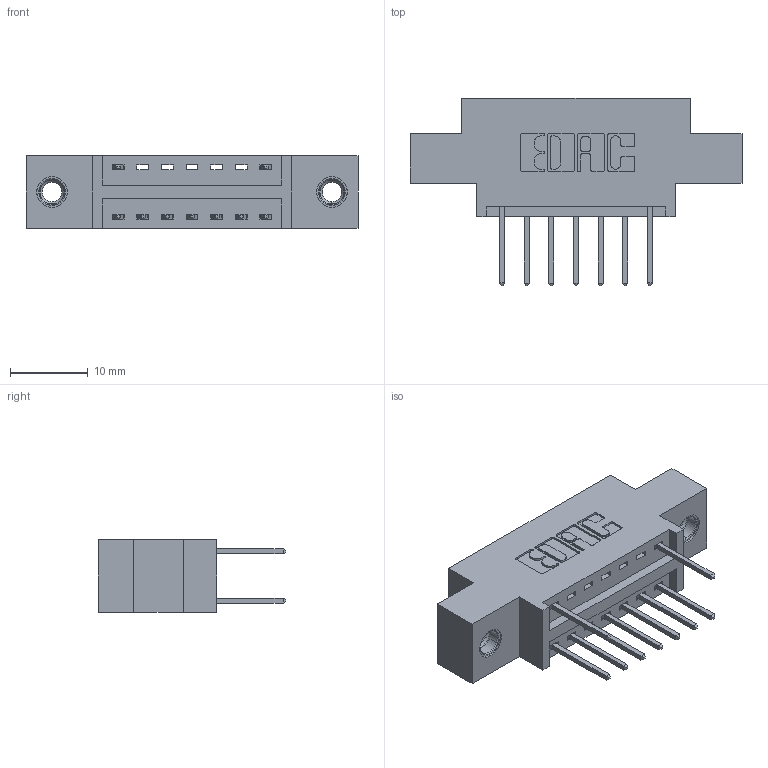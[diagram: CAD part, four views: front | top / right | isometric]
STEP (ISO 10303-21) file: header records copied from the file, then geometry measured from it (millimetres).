
FILE_DESCRIPTION (( 'STEP AP203' ), '1' );
FILE_NAME ('346-014-526-807.STEP', '2018-08-20T01:11:07', ( '' ), ( '' ), 'SwSTEP 2.0', 'SolidWorks 2016', '' );
FILE_SCHEMA (( 'CONFIG_CONTROL_DESIGN' ));
Length unit declared in the file: inch
Products named in the file (4): 346 Part_0.170 Offset - 0.156 Dia-TI; 345-292-001_345-293-126; 345-250-001_345-250-005-103; 346-014-526-807
Assembly tree (12 placements, depth 2):
  346-014-526-807
    346 Part_0.170 Offset - 0.156 Dia-TI
    345-292-001_345-293-126  x9
    345-250-001_345-250-005-103  x2
Bounding box: 42.8 x 24.13 x 9.4 mm (x, y, z)
Volume: 3703.2 mm3; surface area: 4560.2 mm2
Topology: 12 solids, 12 shells, 684 faces, 1977 edges, 1298 vertices
Faces by surface type: plane 452, cylinder 216, cone 12, torus 4
Entity records: 10456 total; most frequent: CARTESIAN_POINT 1778, ORIENTED_EDGE 1710, DIRECTION 1639, EDGE_CURVE 855, VECTOR 675, LINE 675, VERTEX_POINT 564, AXIS2_PLACEMENT_3D 482
